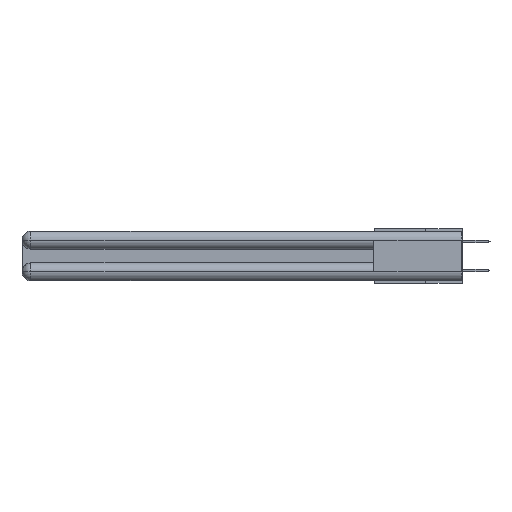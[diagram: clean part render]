
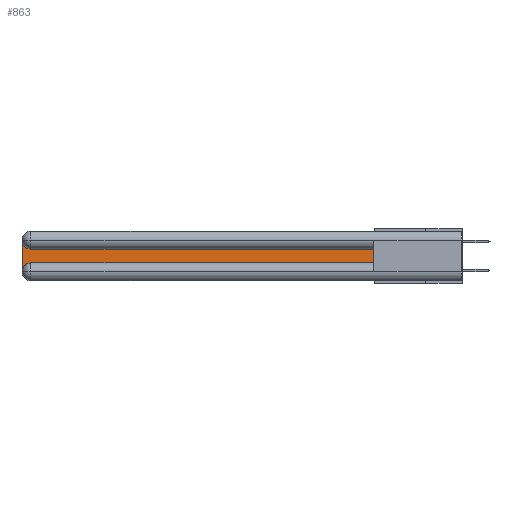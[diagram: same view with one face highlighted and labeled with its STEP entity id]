
A CAD part, left-side view. The second image highlights one B-rep face of the part: STEP entity #863.
In plain terms, the highlighted planar face has unit normal (-1, 0, 0).
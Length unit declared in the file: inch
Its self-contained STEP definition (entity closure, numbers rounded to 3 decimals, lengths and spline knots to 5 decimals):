
#127 = CARTESIAN_POINT ( 'NONE',  ( 0.075, 0.6, -0.2175 ) ) ;
#297 = CARTESIAN_POINT ( 'NONE',  ( 0.075, 2.94, -0.2775 ) ) ;
#863 = ADVANCED_FACE ( 'NONE', ( #18993 ), #4584, .F. ) ;
#1449 = VERTEX_POINT ( 'NONE', #22848 ) ;
#2569 = DIRECTION ( 'NONE',  ( 1., 0., 0. ) ) ;
#2678 = DIRECTION ( 'NONE',  ( 0., 0., -1. ) ) ;
#2933 = CIRCLE ( 'NONE', #15699, 0.06 ) ;
#3412 = DIRECTION ( 'NONE',  ( 0., 0., -1. ) ) ;
#4209 = EDGE_CURVE ( 'NONE', #1449, #11232, #25897, .T. ) ;
#4494 = EDGE_CURVE ( 'NONE', #12916, #22115, #16549, .T. ) ;
#4584 = PLANE ( 'NONE',  #13975 ) ;
#5691 = VECTOR ( 'NONE', #9719, 39.37008 ) ;
#5816 = LINE ( 'NONE', #127, #10676 ) ;
#6778 = CARTESIAN_POINT ( 'NONE',  ( 0.075, 3., -0.2775 ) ) ;
#6969 = CARTESIAN_POINT ( 'NONE',  ( 0.075, 3., -0.1225 ) ) ;
#8229 = DIRECTION ( 'NONE',  ( 0., 1., 0. ) ) ;
#8761 = VECTOR ( 'NONE', #8229, 39.37008 ) ;
#9084 = CARTESIAN_POINT ( 'NONE',  ( 0.075, 2.94, -0.1225 ) ) ;
#9719 = DIRECTION ( 'NONE',  ( 0., -1., 0. ) ) ;
#10196 = DIRECTION ( 'NONE',  ( 1., 0., 0. ) ) ;
#10623 = CARTESIAN_POINT ( 'NONE',  ( 0.075, 2.94, -0.2175 ) ) ;
#10628 = CARTESIAN_POINT ( 'NONE',  ( 0.075, 0.6, -0.1225 ) ) ;
#10676 = VECTOR ( 'NONE', #23655, 39.37008 ) ;
#11232 = VERTEX_POINT ( 'NONE', #9084 ) ;
#11312 = LINE ( 'NONE', #24314, #5691 ) ;
#12256 = DIRECTION ( 'NONE',  ( 0., 0., -1. ) ) ;
#12318 = VERTEX_POINT ( 'NONE', #10623 ) ;
#12916 = VERTEX_POINT ( 'NONE', #21356 ) ;
#12986 = CARTESIAN_POINT ( 'NONE',  ( 0.075, 2.94, -0.0625 ) ) ;
#13032 = EDGE_CURVE ( 'NONE', #12318, #25297, #11312, .T. ) ;
#13975 = AXIS2_PLACEMENT_3D ( 'NONE', #6969, #23633, #2678 ) ;
#15068 = ORIENTED_EDGE ( 'NONE', *, *, #21890, .T. ) ;
#15699 = AXIS2_PLACEMENT_3D ( 'NONE', #12986, #10196, #3412 ) ;
#15958 = CIRCLE ( 'NONE', #20920, 0.06 ) ;
#16549 = LINE ( 'NONE', #22787, #22149 ) ;
#17202 = EDGE_CURVE ( 'NONE', #25297, #1449, #5816, .T. ) ;
#18642 = DIRECTION ( 'NONE',  ( 0., 0., -1. ) ) ;
#18993 = FACE_OUTER_BOUND ( 'NONE', #21564, .T. ) ;
#20920 = AXIS2_PLACEMENT_3D ( 'NONE', #297, #2569, #12256 ) ;
#20957 = EDGE_CURVE ( 'NONE', #11232, #12916, #2933, .T. ) ;
#21356 = CARTESIAN_POINT ( 'NONE',  ( 0.075, 3., -0.0625 ) ) ;
#21564 = EDGE_LOOP ( 'NONE', ( #21738, #28116, #30522, #15068, #29982, #30091 ) ) ;
#21738 = ORIENTED_EDGE ( 'NONE', *, *, #4209, .T. ) ;
#21890 = EDGE_CURVE ( 'NONE', #22115, #12318, #15958, .T. ) ;
#22115 = VERTEX_POINT ( 'NONE', #6778 ) ;
#22149 = VECTOR ( 'NONE', #18642, 39.37008 ) ;
#22787 = CARTESIAN_POINT ( 'NONE',  ( 0.075, 3., -0.2175 ) ) ;
#22848 = CARTESIAN_POINT ( 'NONE',  ( 0.075, 0.6, -0.1225 ) ) ;
#23633 = DIRECTION ( 'NONE',  ( 1., 0., 0. ) ) ;
#23655 = DIRECTION ( 'NONE',  ( 0., 0., 1. ) ) ;
#24314 = CARTESIAN_POINT ( 'NONE',  ( 0.075, 0.6, -0.2175 ) ) ;
#25297 = VERTEX_POINT ( 'NONE', #29954 ) ;
#25897 = LINE ( 'NONE', #10628, #8761 ) ;
#28116 = ORIENTED_EDGE ( 'NONE', *, *, #20957, .T. ) ;
#29954 = CARTESIAN_POINT ( 'NONE',  ( 0.075, 0.6, -0.2175 ) ) ;
#29982 = ORIENTED_EDGE ( 'NONE', *, *, #13032, .T. ) ;
#30091 = ORIENTED_EDGE ( 'NONE', *, *, #17202, .T. ) ;
#30522 = ORIENTED_EDGE ( 'NONE', *, *, #4494, .T. ) ;
